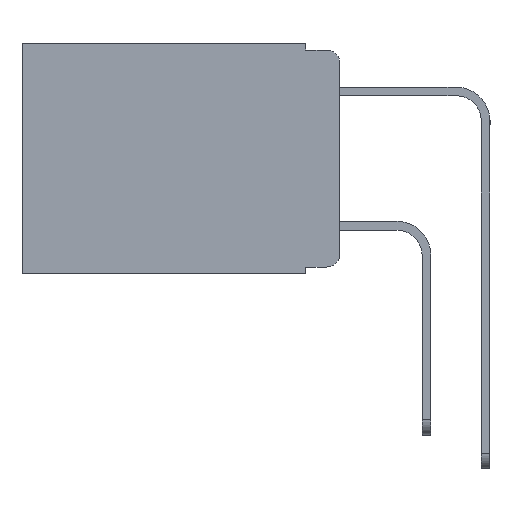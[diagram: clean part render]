
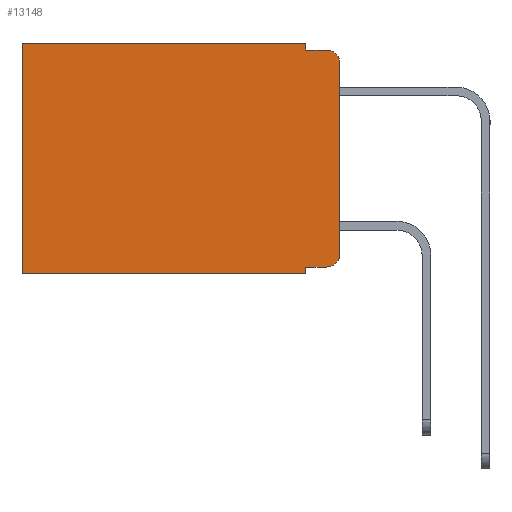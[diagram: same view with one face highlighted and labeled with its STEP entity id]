
A CAD part, left-side view. The second image highlights one B-rep face of the part: STEP entity #13148.
In plain terms, the highlighted planar face has unit normal (-1, 0, 0).
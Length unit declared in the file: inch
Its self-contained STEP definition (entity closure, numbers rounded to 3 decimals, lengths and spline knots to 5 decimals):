
#86 = CARTESIAN_POINT ( 'NONE',  ( 0.298, 0.051, -0.01 ) ) ;
#134 = VERTEX_POINT ( 'NONE', #11759 ) ;
#591 = DIRECTION ( 'NONE',  ( 0., 1., 0. ) ) ;
#630 = LINE ( 'NONE', #6372, #8367 ) ;
#869 = CARTESIAN_POINT ( 'NONE',  ( 0.298, 0.051, 0. ) ) ;
#1136 = EDGE_CURVE ( 'NONE', #2273, #6479, #13800, .T. ) ;
#1387 = CARTESIAN_POINT ( 'NONE',  ( 0.298, 0.051, -0.01 ) ) ;
#1421 = DIRECTION ( 'NONE',  ( 0., 0., -1. ) ) ;
#1458 = EDGE_CURVE ( 'NONE', #14817, #14054, #9385, .T. ) ;
#1721 = VECTOR ( 'NONE', #11426, 39.37008 ) ;
#1854 = CARTESIAN_POINT ( 'NONE',  ( 0.298, 0.051, -0.333 ) ) ;
#2174 = CARTESIAN_POINT ( 'NONE',  ( 0.298, 0., -0.343 ) ) ;
#2215 = PLANE ( 'NONE',  #6818 ) ;
#2218 = VECTOR ( 'NONE', #11586, 39.37008 ) ;
#2272 = CARTESIAN_POINT ( 'NONE',  ( 0.298, 0., 0. ) ) ;
#2273 = VERTEX_POINT ( 'NONE', #7247 ) ;
#2656 = CARTESIAN_POINT ( 'NONE',  ( 0.298, 0., -0.03 ) ) ;
#2741 = DIRECTION ( 'NONE',  ( 0., 0., -1. ) ) ;
#2835 = CARTESIAN_POINT ( 'NONE',  ( 0.298, 0.02, -0.313 ) ) ;
#3446 = VECTOR ( 'NONE', #16060, 39.37008 ) ;
#3474 = DIRECTION ( 'NONE',  ( 0., 0., -1. ) ) ;
#3753 = VERTEX_POINT ( 'NONE', #12398 ) ;
#3818 = CARTESIAN_POINT ( 'NONE',  ( 0.298, 0.02, -0.03 ) ) ;
#3830 = DIRECTION ( 'NONE',  ( 0., 0., -1. ) ) ;
#3937 = DIRECTION ( 'NONE',  ( -1., 0., 0. ) ) ;
#4386 = VERTEX_POINT ( 'NONE', #1854 ) ;
#4419 = CIRCLE ( 'NONE', #7760, 0.02 ) ;
#4558 = CARTESIAN_POINT ( 'NONE',  ( 0.298, 0., -0.313 ) ) ;
#4624 = VECTOR ( 'NONE', #16362, 39.37008 ) ;
#5248 = EDGE_CURVE ( 'NONE', #12693, #6479, #630, .T. ) ;
#6250 = EDGE_CURVE ( 'NONE', #134, #14054, #4419, .T. ) ;
#6372 = CARTESIAN_POINT ( 'NONE',  ( 0.298, 0.473, 0. ) ) ;
#6479 = VERTEX_POINT ( 'NONE', #9080 ) ;
#6818 = AXIS2_PLACEMENT_3D ( 'NONE', #2272, #12727, #3830 ) ;
#6839 = LINE ( 'NONE', #18493, #2218 ) ;
#6951 = DIRECTION ( 'NONE',  ( -1., 0., 0. ) ) ;
#6959 = VERTEX_POINT ( 'NONE', #18526 ) ;
#7247 = CARTESIAN_POINT ( 'NONE',  ( 0.298, 0.051, -0.343 ) ) ;
#7328 = ORIENTED_EDGE ( 'NONE', *, *, #1136, .F. ) ;
#7330 = EDGE_CURVE ( 'NONE', #6959, #18881, #6839, .T. ) ;
#7588 = LINE ( 'NONE', #1387, #3446 ) ;
#7744 = CIRCLE ( 'NONE', #13873, 0.02 ) ;
#7760 = AXIS2_PLACEMENT_3D ( 'NONE', #2835, #3937, #16829 ) ;
#7810 = CARTESIAN_POINT ( 'NONE',  ( 0.298, 0., 0. ) ) ;
#8054 = EDGE_CURVE ( 'NONE', #4386, #134, #8713, .T. ) ;
#8367 = VECTOR ( 'NONE', #1421, 39.37008 ) ;
#8610 = EDGE_CURVE ( 'NONE', #14817, #3753, #7744, .T. ) ;
#8713 = LINE ( 'NONE', #16396, #4624 ) ;
#9080 = CARTESIAN_POINT ( 'NONE',  ( 0.298, 0.473, -0.343 ) ) ;
#9385 = LINE ( 'NONE', #7810, #13147 ) ;
#9617 = ORIENTED_EDGE ( 'NONE', *, *, #1458, .F. ) ;
#11165 = ORIENTED_EDGE ( 'NONE', *, *, #14701, .F. ) ;
#11426 = DIRECTION ( 'NONE',  ( 0., 0., -1. ) ) ;
#11427 = ORIENTED_EDGE ( 'NONE', *, *, #14039, .F. ) ;
#11586 = DIRECTION ( 'NONE',  ( 0., 0., -1. ) ) ;
#11619 = ORIENTED_EDGE ( 'NONE', *, *, #6250, .T. ) ;
#11759 = CARTESIAN_POINT ( 'NONE',  ( 0.298, 0.02, -0.333 ) ) ;
#11809 = EDGE_LOOP ( 'NONE', ( #9617, #14882, #11427, #12664, #18431, #15520, #7328, #11165, #18111, #11619 ) ) ;
#12398 = CARTESIAN_POINT ( 'NONE',  ( 0.298, 0.02, -0.01 ) ) ;
#12569 = VECTOR ( 'NONE', #591, 39.37008 ) ;
#12664 = ORIENTED_EDGE ( 'NONE', *, *, #7330, .F. ) ;
#12693 = VERTEX_POINT ( 'NONE', #14190 ) ;
#12727 = DIRECTION ( 'NONE',  ( 1., 0., 0. ) ) ;
#13147 = VECTOR ( 'NONE', #2741, 39.37008 ) ;
#13148 = ADVANCED_FACE ( 'NONE', ( #18873 ), #2215, .F. ) ;
#13593 = LINE ( 'NONE', #869, #1721 ) ;
#13800 = LINE ( 'NONE', #2174, #17462 ) ;
#13873 = AXIS2_PLACEMENT_3D ( 'NONE', #3818, #6951, #3474 ) ;
#14039 = EDGE_CURVE ( 'NONE', #18881, #3753, #7588, .T. ) ;
#14054 = VERTEX_POINT ( 'NONE', #4558 ) ;
#14190 = CARTESIAN_POINT ( 'NONE',  ( 0.298, 0.473, 0. ) ) ;
#14572 = DIRECTION ( 'NONE',  ( 0., 1., 0. ) ) ;
#14701 = EDGE_CURVE ( 'NONE', #4386, #2273, #13593, .T. ) ;
#14817 = VERTEX_POINT ( 'NONE', #2656 ) ;
#14882 = ORIENTED_EDGE ( 'NONE', *, *, #8610, .T. ) ;
#15256 = CARTESIAN_POINT ( 'NONE',  ( 0.298, 0., 0. ) ) ;
#15520 = ORIENTED_EDGE ( 'NONE', *, *, #5248, .T. ) ;
#16060 = DIRECTION ( 'NONE',  ( 0., -1., 0. ) ) ;
#16222 = LINE ( 'NONE', #15256, #12569 ) ;
#16362 = DIRECTION ( 'NONE',  ( 0., -1., 0. ) ) ;
#16396 = CARTESIAN_POINT ( 'NONE',  ( 0.298, 0.051, -0.333 ) ) ;
#16829 = DIRECTION ( 'NONE',  ( 0., 0., -1. ) ) ;
#17462 = VECTOR ( 'NONE', #14572, 39.37008 ) ;
#17884 = EDGE_CURVE ( 'NONE', #6959, #12693, #16222, .T. ) ;
#18111 = ORIENTED_EDGE ( 'NONE', *, *, #8054, .T. ) ;
#18431 = ORIENTED_EDGE ( 'NONE', *, *, #17884, .T. ) ;
#18493 = CARTESIAN_POINT ( 'NONE',  ( 0.298, 0.051, 0. ) ) ;
#18526 = CARTESIAN_POINT ( 'NONE',  ( 0.298, 0.051, 0. ) ) ;
#18873 = FACE_OUTER_BOUND ( 'NONE', #11809, .T. ) ;
#18881 = VERTEX_POINT ( 'NONE', #86 ) ;
